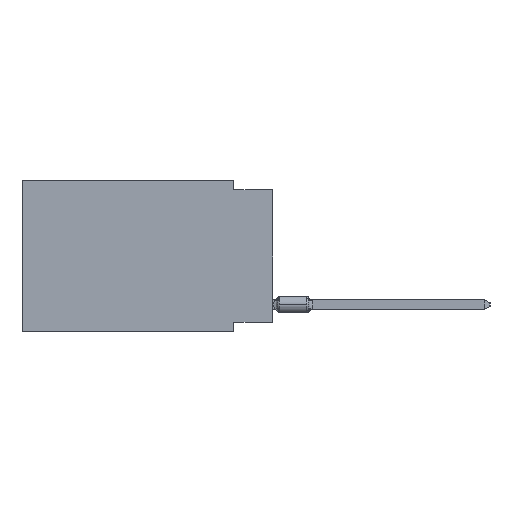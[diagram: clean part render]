
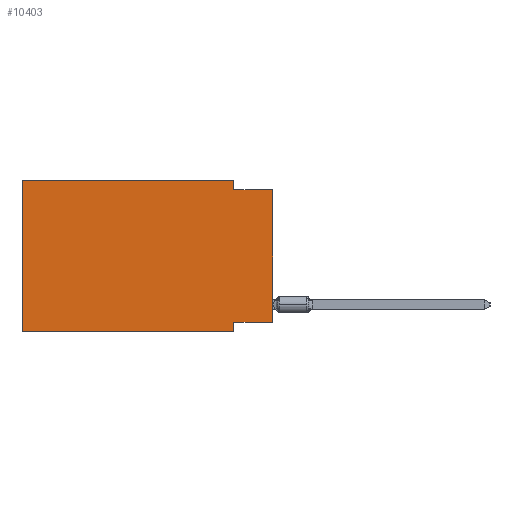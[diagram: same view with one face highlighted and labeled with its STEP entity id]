
A CAD part, left-side view. The second image highlights one B-rep face of the part: STEP entity #10403.
In plain terms, the highlighted planar face has unit normal (-1, 0, 0).
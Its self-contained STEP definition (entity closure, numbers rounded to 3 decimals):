
#514 = PLANE ( 'NONE',  #45682 ) ;
#1603 = VECTOR ( 'NONE', #65105, 1000. ) ;
#2631 = CARTESIAN_POINT ( 'NONE',  ( 0., 0., -0.635 ) ) ;
#2891 = LINE ( 'NONE', #14558, #6064 ) ;
#5038 = CARTESIAN_POINT ( 'NONE',  ( 0., 2.54, -9.271 ) ) ;
#6064 = VECTOR ( 'NONE', #7442, 1000. ) ;
#6733 = CARTESIAN_POINT ( 'NONE',  ( 0., 2.54, -9.906 ) ) ;
#7442 = DIRECTION ( 'NONE',  ( 0., -1., 0. ) ) ;
#7963 = VECTOR ( 'NONE', #47055, 1000. ) ;
#8686 = EDGE_CURVE ( 'NONE', #21453, #44802, #62701, .T. ) ;
#8965 = VECTOR ( 'NONE', #63640, 1000. ) ;
#10403 = ADVANCED_FACE ( 'NONE', ( #69402 ), #514, .F. ) ;
#10565 = ORIENTED_EDGE ( 'NONE', *, *, #73423, .F. ) ;
#10842 = VERTEX_POINT ( 'NONE', #2631 ) ;
#11742 = VERTEX_POINT ( 'NONE', #35011 ) ;
#13223 = CARTESIAN_POINT ( 'NONE',  ( 0., 0., -9.271 ) ) ;
#13610 = ORIENTED_EDGE ( 'NONE', *, *, #23176, .T. ) ;
#14558 = CARTESIAN_POINT ( 'NONE',  ( 0., 16.383, -9.906 ) ) ;
#16886 = ORIENTED_EDGE ( 'NONE', *, *, #34176, .F. ) ;
#21453 = VERTEX_POINT ( 'NONE', #64578 ) ;
#22662 = EDGE_LOOP ( 'NONE', ( #50439, #16886, #60496, #23583, #34327, #13610, #10565, #26660 ) ) ;
#23176 = EDGE_CURVE ( 'NONE', #11742, #50783, #2891, .T. ) ;
#23471 = DIRECTION ( 'NONE',  ( 0., 0., -1. ) ) ;
#23583 = ORIENTED_EDGE ( 'NONE', *, *, #49852, .F. ) ;
#24171 = CARTESIAN_POINT ( 'NONE',  ( 0., 16.383, 0. ) ) ;
#26660 = ORIENTED_EDGE ( 'NONE', *, *, #59058, .F. ) ;
#26853 = CARTESIAN_POINT ( 'NONE',  ( 0., 2.54, -9.906 ) ) ;
#28396 = DIRECTION ( 'NONE',  ( 1., 0., 0. ) ) ;
#28406 = VERTEX_POINT ( 'NONE', #33843 ) ;
#33097 = VECTOR ( 'NONE', #42232, 1000. ) ;
#33403 = CARTESIAN_POINT ( 'NONE',  ( 0., 2.54, -0.635 ) ) ;
#33843 = CARTESIAN_POINT ( 'NONE',  ( 0., 16.383, 0. ) ) ;
#34176 = EDGE_CURVE ( 'NONE', #44802, #10842, #41046, .T. ) ;
#34327 = ORIENTED_EDGE ( 'NONE', *, *, #66538, .F. ) ;
#35011 = CARTESIAN_POINT ( 'NONE',  ( 0., 16.383, -9.906 ) ) ;
#35071 = LINE ( 'NONE', #24171, #33097 ) ;
#35362 = CARTESIAN_POINT ( 'NONE',  ( 0., 0., -9.271 ) ) ;
#36883 = VECTOR ( 'NONE', #65162, 1000. ) ;
#41046 = LINE ( 'NONE', #64014, #7963 ) ;
#41286 = VERTEX_POINT ( 'NONE', #35362 ) ;
#41805 = CARTESIAN_POINT ( 'NONE',  ( 0., 0., 0. ) ) ;
#42232 = DIRECTION ( 'NONE',  ( 0., -1., 0. ) ) ;
#44802 = VERTEX_POINT ( 'NONE', #33403 ) ;
#45542 = EDGE_CURVE ( 'NONE', #41286, #10842, #69675, .T. ) ;
#45682 = AXIS2_PLACEMENT_3D ( 'NONE', #68294, #28396, #23471 ) ;
#46641 = CARTESIAN_POINT ( 'NONE',  ( 0., 16.383, 0. ) ) ;
#47055 = DIRECTION ( 'NONE',  ( 0., -1., 0. ) ) ;
#49852 = EDGE_CURVE ( 'NONE', #28406, #21453, #35071, .T. ) ;
#50439 = ORIENTED_EDGE ( 'NONE', *, *, #45542, .T. ) ;
#50783 = VERTEX_POINT ( 'NONE', #26853 ) ;
#51543 = VECTOR ( 'NONE', #69842, 1000. ) ;
#52139 = CARTESIAN_POINT ( 'NONE',  ( 0., 2.54, 0. ) ) ;
#53382 = DIRECTION ( 'NONE',  ( 0., 0., -1. ) ) ;
#59058 = EDGE_CURVE ( 'NONE', #41286, #69618, #64781, .T. ) ;
#59441 = LINE ( 'NONE', #46641, #1603 ) ;
#60496 = ORIENTED_EDGE ( 'NONE', *, *, #8686, .F. ) ;
#62701 = LINE ( 'NONE', #52139, #51543 ) ;
#63640 = DIRECTION ( 'NONE',  ( 0., 0., 1. ) ) ;
#64014 = CARTESIAN_POINT ( 'NONE',  ( 0., 0., -0.635 ) ) ;
#64578 = CARTESIAN_POINT ( 'NONE',  ( 0., 2.54, 0. ) ) ;
#64781 = LINE ( 'NONE', #13223, #36883 ) ;
#65105 = DIRECTION ( 'NONE',  ( 0., 0., 1. ) ) ;
#65162 = DIRECTION ( 'NONE',  ( 0., 1., 0. ) ) ;
#66538 = EDGE_CURVE ( 'NONE', #11742, #28406, #59441, .T. ) ;
#68294 = CARTESIAN_POINT ( 'NONE',  ( 0., 16.383, 0. ) ) ;
#69402 = FACE_OUTER_BOUND ( 'NONE', #22662, .T. ) ;
#69618 = VERTEX_POINT ( 'NONE', #5038 ) ;
#69675 = LINE ( 'NONE', #41805, #8965 ) ;
#69842 = DIRECTION ( 'NONE',  ( 0., 0., -1. ) ) ;
#70310 = LINE ( 'NONE', #6733, #70859 ) ;
#70859 = VECTOR ( 'NONE', #53382, 1000. ) ;
#73423 = EDGE_CURVE ( 'NONE', #69618, #50783, #70310, .T. ) ;
